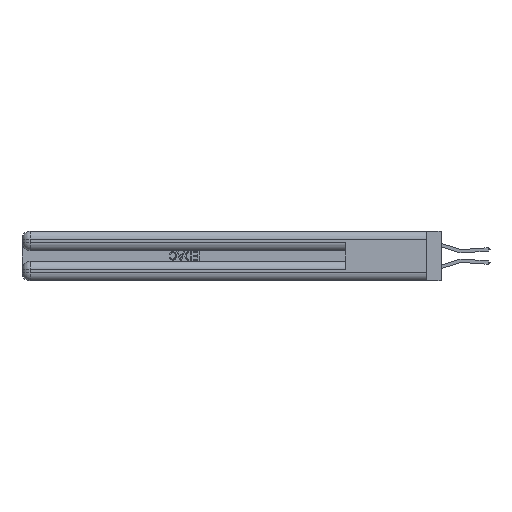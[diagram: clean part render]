
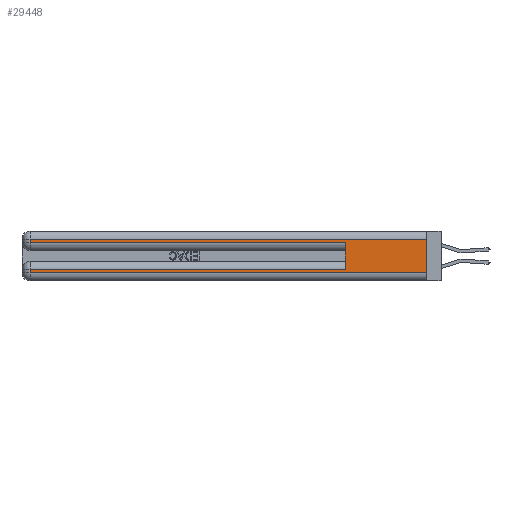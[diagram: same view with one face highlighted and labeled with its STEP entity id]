
A CAD part, left-side view. The second image highlights one B-rep face of the part: STEP entity #29448.
In plain terms, the highlighted planar face has unit normal (-1, 0, 0).
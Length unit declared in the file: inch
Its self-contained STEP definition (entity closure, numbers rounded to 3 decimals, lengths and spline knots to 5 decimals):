
#59 = VECTOR ( 'NONE', #11735, 39.37008 ) ;
#220 = EDGE_CURVE ( 'NONE', #12853, #27944, #8323, .T. ) ;
#589 = VECTOR ( 'NONE', #31255, 39.37008 ) ;
#716 = ORIENTED_EDGE ( 'NONE', *, *, #2134, .T. ) ;
#1145 = VERTEX_POINT ( 'NONE', #18860 ) ;
#1921 = CARTESIAN_POINT ( 'NONE',  ( 0., 2.94, 0.37 ) ) ;
#2058 = DIRECTION ( 'NONE',  ( 0., 0., -1. ) ) ;
#2134 = EDGE_CURVE ( 'NONE', #1145, #32781, #10168, .T. ) ;
#3640 = VECTOR ( 'NONE', #37339, 39.37008 ) ;
#6228 = CARTESIAN_POINT ( 'NONE',  ( 0., 0., 0.085 ) ) ;
#6374 = ORIENTED_EDGE ( 'NONE', *, *, #20407, .T. ) ;
#6472 = VERTEX_POINT ( 'NONE', #31278 ) ;
#8323 = LINE ( 'NONE', #23890, #10334 ) ;
#8525 = CARTESIAN_POINT ( 'NONE',  ( 0., 0., 0.06 ) ) ;
#9378 = CARTESIAN_POINT ( 'NONE',  ( 0., 0., 0.37 ) ) ;
#9403 = DIRECTION ( 'NONE',  ( 0., 1., 0. ) ) ;
#9973 = EDGE_CURVE ( 'NONE', #6472, #10232, #17565, .T. ) ;
#10168 = LINE ( 'NONE', #15943, #3640 ) ;
#10232 = VERTEX_POINT ( 'NONE', #26688 ) ;
#10334 = VECTOR ( 'NONE', #14630, 39.37008 ) ;
#11095 = LINE ( 'NONE', #1921, #26541 ) ;
#11735 = DIRECTION ( 'NONE',  ( 0., -1., 0. ) ) ;
#11783 = DIRECTION ( 'NONE',  ( 0., 0., -1. ) ) ;
#12364 = CARTESIAN_POINT ( 'NONE',  ( 0., 2.94, 0.06 ) ) ;
#12788 = ORIENTED_EDGE ( 'NONE', *, *, #220, .T. ) ;
#12853 = VERTEX_POINT ( 'NONE', #16906 ) ;
#13397 = VERTEX_POINT ( 'NONE', #25698 ) ;
#14393 = VERTEX_POINT ( 'NONE', #36351 ) ;
#14630 = DIRECTION ( 'NONE',  ( 0., 1., 0. ) ) ;
#15943 = CARTESIAN_POINT ( 'NONE',  ( 0., 2.94, 0.37 ) ) ;
#16906 = CARTESIAN_POINT ( 'NONE',  ( 0., 0., 0.31 ) ) ;
#17078 = LINE ( 'NONE', #8525, #59 ) ;
#17565 = LINE ( 'NONE', #19082, #589 ) ;
#18860 = CARTESIAN_POINT ( 'NONE',  ( 0., 2.94, 0.085 ) ) ;
#19082 = CARTESIAN_POINT ( 'NONE',  ( 0., 0.6, 0.145 ) ) ;
#20407 = EDGE_CURVE ( 'NONE', #13397, #10232, #21810, .T. ) ;
#20718 = VECTOR ( 'NONE', #9403, 39.37008 ) ;
#21066 = AXIS2_PLACEMENT_3D ( 'NONE', #27149, #36221, #11783 ) ;
#21810 = LINE ( 'NONE', #37258, #38060 ) ;
#22041 = DIRECTION ( 'NONE',  ( 0., -1., 0. ) ) ;
#22932 = ORIENTED_EDGE ( 'NONE', *, *, #9973, .F. ) ;
#23215 = CARTESIAN_POINT ( 'NONE',  ( 0., 2.94, 0.31 ) ) ;
#23890 = CARTESIAN_POINT ( 'NONE',  ( 0., 0., 0.31 ) ) ;
#24867 = ORIENTED_EDGE ( 'NONE', *, *, #33456, .T. ) ;
#25556 = EDGE_CURVE ( 'NONE', #12853, #14393, #35398, .T. ) ;
#25698 = CARTESIAN_POINT ( 'NONE',  ( 0., 2.94, 0.285 ) ) ;
#25825 = EDGE_LOOP ( 'NONE', ( #28198, #12788, #38234, #6374, #22932, #24867, #716, #35845 ) ) ;
#26541 = VECTOR ( 'NONE', #2058, 39.37008 ) ;
#26688 = CARTESIAN_POINT ( 'NONE',  ( 0., 0.6, 0.285 ) ) ;
#27149 = CARTESIAN_POINT ( 'NONE',  ( 0., 0., 0.37 ) ) ;
#27944 = VERTEX_POINT ( 'NONE', #23215 ) ;
#28198 = ORIENTED_EDGE ( 'NONE', *, *, #25556, .F. ) ;
#28247 = VECTOR ( 'NONE', #30974, 39.37008 ) ;
#29448 = ADVANCED_FACE ( 'NONE', ( #40060 ), #30217, .F. ) ;
#30116 = EDGE_CURVE ( 'NONE', #32781, #14393, #17078, .T. ) ;
#30217 = PLANE ( 'NONE',  #21066 ) ;
#30974 = DIRECTION ( 'NONE',  ( 0., 0., -1. ) ) ;
#31255 = DIRECTION ( 'NONE',  ( 0., 0., 1. ) ) ;
#31278 = CARTESIAN_POINT ( 'NONE',  ( 0., 0.6, 0.085 ) ) ;
#32781 = VERTEX_POINT ( 'NONE', #12364 ) ;
#33456 = EDGE_CURVE ( 'NONE', #6472, #1145, #36941, .T. ) ;
#35398 = LINE ( 'NONE', #9378, #28247 ) ;
#35845 = ORIENTED_EDGE ( 'NONE', *, *, #30116, .T. ) ;
#36019 = EDGE_CURVE ( 'NONE', #27944, #13397, #11095, .T. ) ;
#36221 = DIRECTION ( 'NONE',  ( 1., 0., 0. ) ) ;
#36351 = CARTESIAN_POINT ( 'NONE',  ( 0., 0., 0.06 ) ) ;
#36941 = LINE ( 'NONE', #6228, #20718 ) ;
#37258 = CARTESIAN_POINT ( 'NONE',  ( 0., 0., 0.285 ) ) ;
#37339 = DIRECTION ( 'NONE',  ( 0., 0., -1. ) ) ;
#38060 = VECTOR ( 'NONE', #22041, 39.37008 ) ;
#38234 = ORIENTED_EDGE ( 'NONE', *, *, #36019, .T. ) ;
#40060 = FACE_OUTER_BOUND ( 'NONE', #25825, .T. ) ;
